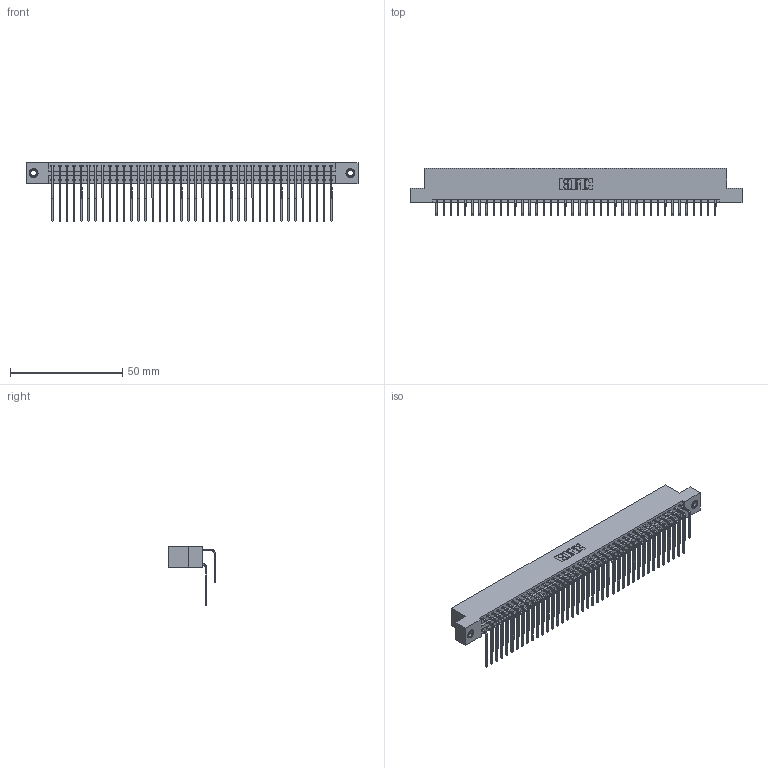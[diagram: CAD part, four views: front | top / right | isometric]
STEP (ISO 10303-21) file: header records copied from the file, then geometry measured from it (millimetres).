
FILE_DESCRIPTION (( 'STEP AP203' ), '1' );
FILE_NAME ('346-080-559-207.STEP', '2022-05-25T16:39:58', ( '' ), ( '' ), 'SwSTEP 2.0', 'SolidWorks 2020', '' );
FILE_SCHEMA (( 'CONFIG_CONTROL_DESIGN' ));
Length unit declared in the file: inch
Products named in the file (5): 346 Part_Flush Mounting Lugs - 0.156 Dia-TI; 346-080-559-207; 345-292-001_558 559 Tail - 1; 345-250-001_345-250-005-103; 345-292-001_559 Tail - 2
Assembly tree (83 placements, depth 2):
  346-080-559-207
    346 Part_Flush Mounting Lugs - 0.156 Dia-TI
    345-292-001_558 559 Tail - 1  x40
    345-292-001_559 Tail - 2  x40
    345-250-001_345-250-005-103  x2
Bounding box: 147.57 x 20.89 x 26.16 mm (x, y, z)
Volume: 14822.7 mm3; surface area: 22591.2 mm2
Topology: 83 solids, 83 shells, 4502 faces, 13345 edges, 8782 vertices
Faces by surface type: plane 3068, cylinder 1418, cone 12, torus 4
Entity records: 29344 total; most frequent: CARTESIAN_POINT 4874, ORIENTED_EDGE 4750, DIRECTION 4345, EDGE_CURVE 2375, LINE 2023, VECTOR 2023, VERTEX_POINT 1576, AXIS2_PLACEMENT_3D 1161
